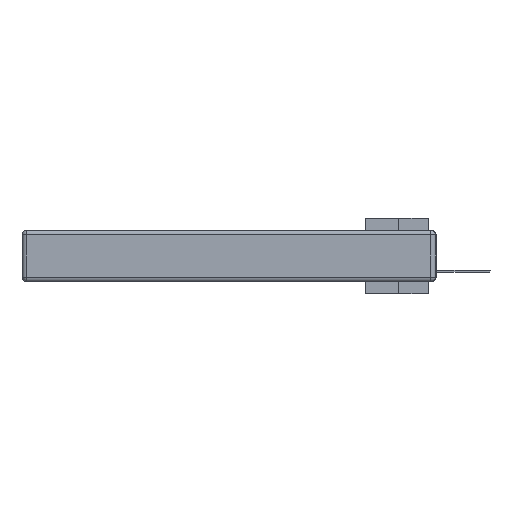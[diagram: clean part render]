
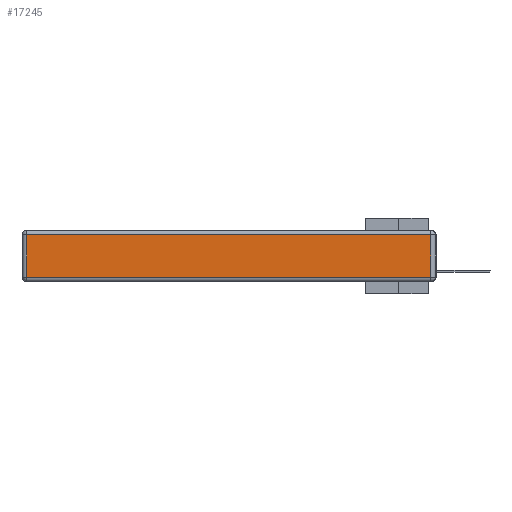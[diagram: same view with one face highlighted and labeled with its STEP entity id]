
A CAD part, left-side view. The second image highlights one B-rep face of the part: STEP entity #17245.
In plain terms, the highlighted planar face has unit normal (-1, 0, 0).
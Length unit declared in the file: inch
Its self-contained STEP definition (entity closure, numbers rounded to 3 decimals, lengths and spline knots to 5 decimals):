
#415 = CARTESIAN_POINT ( 'NONE',  ( 0., 2.72, -0.03 ) ) ;
#629 = CARTESIAN_POINT ( 'NONE',  ( 0., 2.75, -0.03 ) ) ;
#653 = CARTESIAN_POINT ( 'NONE',  ( 0., 0.03, -0.03 ) ) ;
#3234 = LINE ( 'NONE', #3586, #8613 ) ;
#3586 = CARTESIAN_POINT ( 'NONE',  ( 0., 0.03, -0.343 ) ) ;
#4819 = EDGE_LOOP ( 'NONE', ( #29565, #33816, #12410, #35027 ) ) ;
#5498 = DIRECTION ( 'NONE',  ( 0., 0., -1. ) ) ;
#6958 = AXIS2_PLACEMENT_3D ( 'NONE', #12671, #31874, #32406 ) ;
#8045 = LINE ( 'NONE', #35736, #24642 ) ;
#8613 = VECTOR ( 'NONE', #25671, 39.37008 ) ;
#9246 = EDGE_CURVE ( 'NONE', #10709, #22357, #29754, .T. ) ;
#9259 = EDGE_CURVE ( 'NONE', #22357, #23794, #8045, .T. ) ;
#10709 = VERTEX_POINT ( 'NONE', #415 ) ;
#12410 = ORIENTED_EDGE ( 'NONE', *, *, #19439, .T. ) ;
#12462 = VECTOR ( 'NONE', #5498, 39.37008 ) ;
#12671 = CARTESIAN_POINT ( 'NONE',  ( 0., 0., -0.343 ) ) ;
#13686 = EDGE_CURVE ( 'NONE', #23794, #30474, #3234, .T. ) ;
#13764 = CARTESIAN_POINT ( 'NONE',  ( 0., 2.72, -0.313 ) ) ;
#15760 = FACE_OUTER_BOUND ( 'NONE', #4819, .T. ) ;
#17245 = ADVANCED_FACE ( 'NONE', ( #15760 ), #28993, .T. ) ;
#18734 = DIRECTION ( 'NONE',  ( 0., -1., 0. ) ) ;
#19439 = EDGE_CURVE ( 'NONE', #30474, #10709, #25447, .T. ) ;
#22357 = VERTEX_POINT ( 'NONE', #13764 ) ;
#23794 = VERTEX_POINT ( 'NONE', #28310 ) ;
#24642 = VECTOR ( 'NONE', #18734, 39.37008 ) ;
#25447 = LINE ( 'NONE', #629, #26159 ) ;
#25671 = DIRECTION ( 'NONE',  ( 0., 0., 1. ) ) ;
#26159 = VECTOR ( 'NONE', #33929, 39.37008 ) ;
#28310 = CARTESIAN_POINT ( 'NONE',  ( 0., 0.03, -0.313 ) ) ;
#28993 = PLANE ( 'NONE',  #6958 ) ;
#29565 = ORIENTED_EDGE ( 'NONE', *, *, #9259, .T. ) ;
#29754 = LINE ( 'NONE', #35374, #12462 ) ;
#30474 = VERTEX_POINT ( 'NONE', #653 ) ;
#31874 = DIRECTION ( 'NONE',  ( -1., 0., 0. ) ) ;
#32406 = DIRECTION ( 'NONE',  ( 0., 0., 1. ) ) ;
#33816 = ORIENTED_EDGE ( 'NONE', *, *, #13686, .T. ) ;
#33929 = DIRECTION ( 'NONE',  ( 0., 1., 0. ) ) ;
#35027 = ORIENTED_EDGE ( 'NONE', *, *, #9246, .T. ) ;
#35374 = CARTESIAN_POINT ( 'NONE',  ( 0., 2.72, -0.343 ) ) ;
#35736 = CARTESIAN_POINT ( 'NONE',  ( 0., 0., -0.313 ) ) ;
